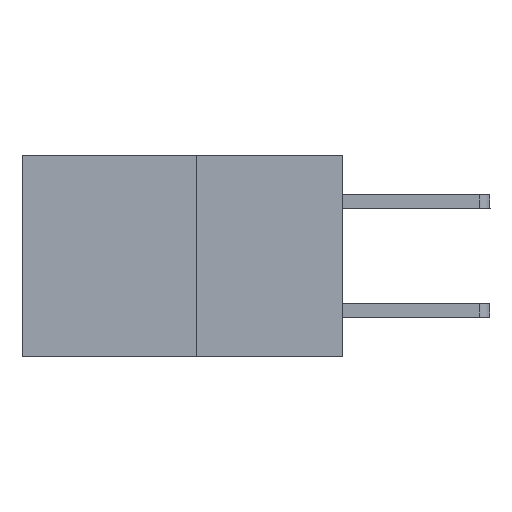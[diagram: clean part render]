
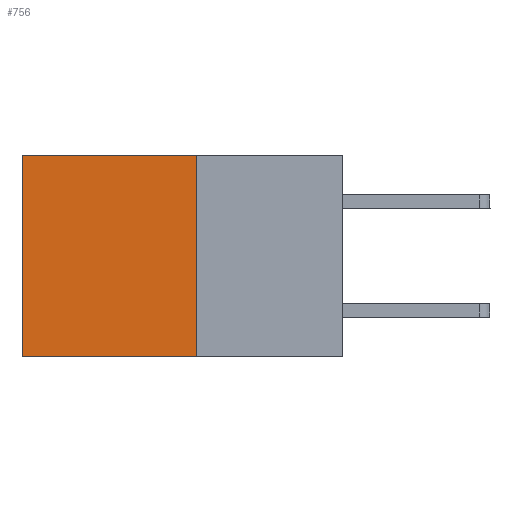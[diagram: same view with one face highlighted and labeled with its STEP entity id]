
A CAD part, left-side view. The second image highlights one B-rep face of the part: STEP entity #756.
In plain terms, the highlighted planar face has unit normal (-1, 0, 0).
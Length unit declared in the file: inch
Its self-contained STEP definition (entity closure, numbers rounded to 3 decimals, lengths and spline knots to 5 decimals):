
#202 = VERTEX_POINT ( 'NONE', #10310 ) ;
#654 = DIRECTION ( 'NONE',  ( 0., 1., 0. ) ) ;
#756 = ADVANCED_FACE ( 'NONE', ( #3794 ), #6921, .F. ) ;
#1032 = EDGE_CURVE ( 'NONE', #1660, #4972, #1092, .T. ) ;
#1092 = LINE ( 'NONE', #2275, #3649 ) ;
#1399 = CARTESIAN_POINT ( 'NONE',  ( 0.277, 0.27, -0.37 ) ) ;
#1660 = VERTEX_POINT ( 'NONE', #1399 ) ;
#2157 = LINE ( 'NONE', #5393, #6826 ) ;
#2247 = EDGE_CURVE ( 'NONE', #202, #1660, #8967, .T. ) ;
#2275 = CARTESIAN_POINT ( 'NONE',  ( 0.277, 0.27, -0.37 ) ) ;
#2294 = LINE ( 'NONE', #3256, #6945 ) ;
#2582 = DIRECTION ( 'NONE',  ( 0., 0., -1. ) ) ;
#2857 = EDGE_CURVE ( 'NONE', #3594, #4972, #2294, .T. ) ;
#3115 = DIRECTION ( 'NONE',  ( 0., 0., -1. ) ) ;
#3256 = CARTESIAN_POINT ( 'NONE',  ( 0.277, 0.59, -0.37 ) ) ;
#3563 = CARTESIAN_POINT ( 'NONE',  ( 0.277, 0.59, 0. ) ) ;
#3594 = VERTEX_POINT ( 'NONE', #3563 ) ;
#3649 = VECTOR ( 'NONE', #6560, 39.37008 ) ;
#3794 = FACE_OUTER_BOUND ( 'NONE', #6496, .T. ) ;
#4972 = VERTEX_POINT ( 'NONE', #7269 ) ;
#5386 = ORIENTED_EDGE ( 'NONE', *, *, #2247, .F. ) ;
#5393 = CARTESIAN_POINT ( 'NONE',  ( 0.277, 0.27, 0. ) ) ;
#5579 = EDGE_CURVE ( 'NONE', #202, #3594, #2157, .T. ) ;
#5928 = DIRECTION ( 'NONE',  ( 1., 0., 0. ) ) ;
#6110 = AXIS2_PLACEMENT_3D ( 'NONE', #9781, #5928, #2582 ) ;
#6496 = EDGE_LOOP ( 'NONE', ( #11675, #9130, #5386, #11967 ) ) ;
#6560 = DIRECTION ( 'NONE',  ( 0., 1., 0. ) ) ;
#6826 = VECTOR ( 'NONE', #654, 39.37008 ) ;
#6921 = PLANE ( 'NONE',  #6110 ) ;
#6945 = VECTOR ( 'NONE', #3115, 39.37008 ) ;
#7269 = CARTESIAN_POINT ( 'NONE',  ( 0.277, 0.59, -0.37 ) ) ;
#8967 = LINE ( 'NONE', #10333, #9247 ) ;
#9130 = ORIENTED_EDGE ( 'NONE', *, *, #1032, .F. ) ;
#9247 = VECTOR ( 'NONE', #10359, 39.37008 ) ;
#9781 = CARTESIAN_POINT ( 'NONE',  ( 0.277, 0.27, -0.37 ) ) ;
#10310 = CARTESIAN_POINT ( 'NONE',  ( 0.277, 0.27, 0. ) ) ;
#10333 = CARTESIAN_POINT ( 'NONE',  ( 0.277, 0.27, -0.37 ) ) ;
#10359 = DIRECTION ( 'NONE',  ( 0., 0., -1. ) ) ;
#11675 = ORIENTED_EDGE ( 'NONE', *, *, #2857, .T. ) ;
#11967 = ORIENTED_EDGE ( 'NONE', *, *, #5579, .T. ) ;
